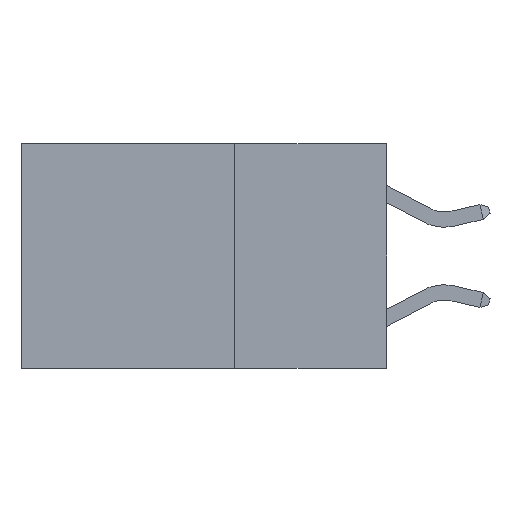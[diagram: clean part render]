
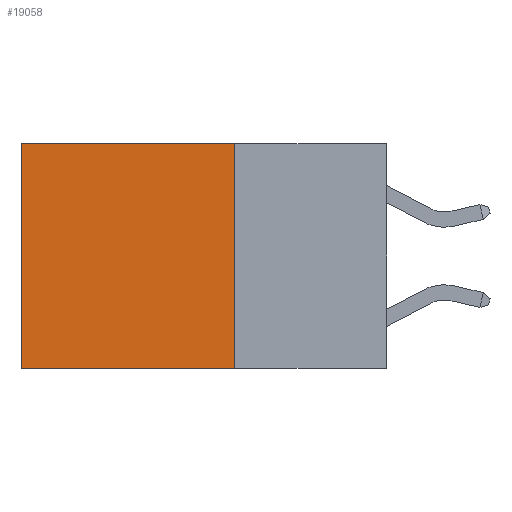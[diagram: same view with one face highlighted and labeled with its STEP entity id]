
A CAD part, left-side view. The second image highlights one B-rep face of the part: STEP entity #19058.
In plain terms, the highlighted planar face has unit normal (-1, 0, 0).
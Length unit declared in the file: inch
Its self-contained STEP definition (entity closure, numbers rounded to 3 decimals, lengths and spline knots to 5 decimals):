
#550 = VERTEX_POINT ( 'NONE', #17883 ) ;
#987 = LINE ( 'NONE', #7546, #5137 ) ;
#2892 = FACE_OUTER_BOUND ( 'NONE', #18037, .T. ) ;
#2903 = CARTESIAN_POINT ( 'NONE',  ( 0.2625, 0.6, 0. ) ) ;
#3121 = DIRECTION ( 'NONE',  ( 1., 0., 0. ) ) ;
#3328 = CARTESIAN_POINT ( 'NONE',  ( 0.2625, 0.25, 0. ) ) ;
#3456 = AXIS2_PLACEMENT_3D ( 'NONE', #3328, #3121, #15229 ) ;
#3822 = VERTEX_POINT ( 'NONE', #20015 ) ;
#4682 = ORIENTED_EDGE ( 'NONE', *, *, #15922, .T. ) ;
#4802 = CARTESIAN_POINT ( 'NONE',  ( 0.2625, 0.6, -0.37 ) ) ;
#5137 = VECTOR ( 'NONE', #16271, 39.37008 ) ;
#6266 = EDGE_CURVE ( 'NONE', #6349, #7023, #21264, .T. ) ;
#6349 = VERTEX_POINT ( 'NONE', #2903 ) ;
#7023 = VERTEX_POINT ( 'NONE', #4802 ) ;
#7546 = CARTESIAN_POINT ( 'NONE',  ( 0.2625, 0.25, 0. ) ) ;
#8145 = CARTESIAN_POINT ( 'NONE',  ( 0.2625, 0.25, 0. ) ) ;
#9584 = CARTESIAN_POINT ( 'NONE',  ( 0.2625, 0.6, 0. ) ) ;
#10462 = EDGE_CURVE ( 'NONE', #550, #3822, #15398, .T. ) ;
#11300 = ORIENTED_EDGE ( 'NONE', *, *, #14764, .F. ) ;
#11340 = ORIENTED_EDGE ( 'NONE', *, *, #10462, .F. ) ;
#11388 = ORIENTED_EDGE ( 'NONE', *, *, #6266, .T. ) ;
#11397 = CARTESIAN_POINT ( 'NONE',  ( 0.2625, 0.25, -0.37 ) ) ;
#11522 = DIRECTION ( 'NONE',  ( 0., 1., 0. ) ) ;
#12374 = VECTOR ( 'NONE', #11522, 39.37008 ) ;
#13431 = LINE ( 'NONE', #11397, #12374 ) ;
#14764 = EDGE_CURVE ( 'NONE', #3822, #7023, #13431, .T. ) ;
#15229 = DIRECTION ( 'NONE',  ( 0., 0., -1. ) ) ;
#15398 = LINE ( 'NONE', #8145, #19705 ) ;
#15922 = EDGE_CURVE ( 'NONE', #550, #6349, #987, .T. ) ;
#16271 = DIRECTION ( 'NONE',  ( 0., 1., 0. ) ) ;
#16651 = DIRECTION ( 'NONE',  ( 0., 0., -1. ) ) ;
#17883 = CARTESIAN_POINT ( 'NONE',  ( 0.2625, 0.25, 0. ) ) ;
#18037 = EDGE_LOOP ( 'NONE', ( #11388, #11300, #11340, #4682 ) ) ;
#18199 = DIRECTION ( 'NONE',  ( 0., 0., -1. ) ) ;
#18654 = PLANE ( 'NONE',  #3456 ) ;
#19058 = ADVANCED_FACE ( 'NONE', ( #2892 ), #18654, .F. ) ;
#19705 = VECTOR ( 'NONE', #16651, 39.37008 ) ;
#19760 = VECTOR ( 'NONE', #18199, 39.37008 ) ;
#20015 = CARTESIAN_POINT ( 'NONE',  ( 0.2625, 0.25, -0.37 ) ) ;
#21264 = LINE ( 'NONE', #9584, #19760 ) ;
